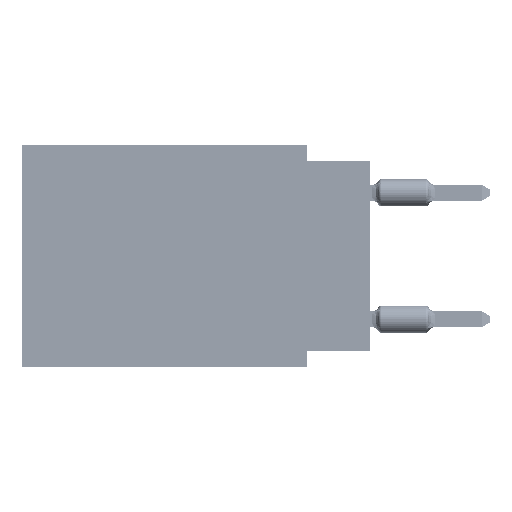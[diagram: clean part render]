
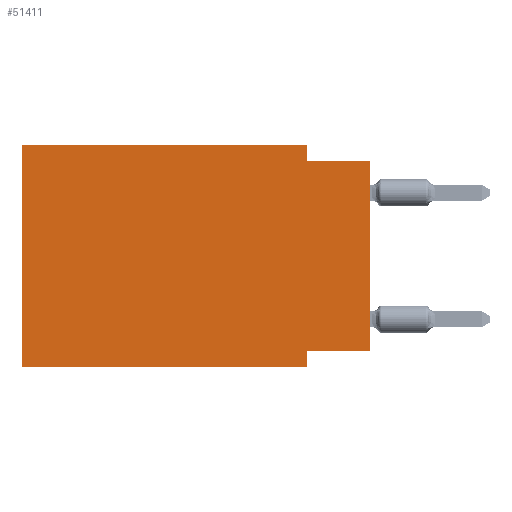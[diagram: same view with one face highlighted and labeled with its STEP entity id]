
A CAD part, left-side view. The second image highlights one B-rep face of the part: STEP entity #51411.
In plain terms, the highlighted planar face has unit normal (-1, 0, 0).
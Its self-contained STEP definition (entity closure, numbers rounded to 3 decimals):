
#2846 = DIRECTION ( 'NONE',  ( 0., 0., -1. ) ) ;
#4109 = DIRECTION ( 'NONE',  ( 0., 0., 1. ) ) ;
#4521 = LINE ( 'NONE', #8218, #76944 ) ;
#4788 = CARTESIAN_POINT ( 'NONE',  ( 0., 0., -0.635 ) ) ;
#6549 = CARTESIAN_POINT ( 'NONE',  ( 0., 2.54, 0. ) ) ;
#6938 = PLANE ( 'NONE',  #75729 ) ;
#8218 = CARTESIAN_POINT ( 'NONE',  ( 0., 2.54, 0. ) ) ;
#8310 = VECTOR ( 'NONE', #4109, 1000. ) ;
#9479 = ORIENTED_EDGE ( 'NONE', *, *, #40379, .T. ) ;
#9956 = VERTEX_POINT ( 'NONE', #65467 ) ;
#10129 = VECTOR ( 'NONE', #35902, 1000. ) ;
#10165 = ORIENTED_EDGE ( 'NONE', *, *, #57154, .F. ) ;
#11423 = VERTEX_POINT ( 'NONE', #36350 ) ;
#12051 = EDGE_CURVE ( 'NONE', #71696, #49729, #40936, .T. ) ;
#18759 = VECTOR ( 'NONE', #71883, 1000. ) ;
#18828 = CARTESIAN_POINT ( 'NONE',  ( 0., 0., 0. ) ) ;
#19589 = LINE ( 'NONE', #58834, #8310 ) ;
#22375 = CARTESIAN_POINT ( 'NONE',  ( 0., 13.97, -8.89 ) ) ;
#23101 = LINE ( 'NONE', #53623, #18759 ) ;
#23820 = VERTEX_POINT ( 'NONE', #47737 ) ;
#26851 = EDGE_CURVE ( 'NONE', #49729, #57755, #4521, .T. ) ;
#28266 = CARTESIAN_POINT ( 'NONE',  ( 0., 13.97, 0. ) ) ;
#31113 = CARTESIAN_POINT ( 'NONE',  ( 0., 13.97, 0. ) ) ;
#32017 = DIRECTION ( 'NONE',  ( 0., -1., 0. ) ) ;
#33629 = CARTESIAN_POINT ( 'NONE',  ( 0., 2.54, -0.635 ) ) ;
#34248 = EDGE_CURVE ( 'NONE', #57755, #11423, #39673, .T. ) ;
#35003 = DIRECTION ( 'NONE',  ( 0., -1., 0. ) ) ;
#35902 = DIRECTION ( 'NONE',  ( 0., 0., 1. ) ) ;
#36350 = CARTESIAN_POINT ( 'NONE',  ( 0., 0., -0.635 ) ) ;
#37305 = LINE ( 'NONE', #38091, #49177 ) ;
#37329 = EDGE_CURVE ( 'NONE', #37973, #60269, #49864, .T. ) ;
#37948 = CARTESIAN_POINT ( 'NONE',  ( 0., 13.97, -8.89 ) ) ;
#37973 = VERTEX_POINT ( 'NONE', #22375 ) ;
#38091 = CARTESIAN_POINT ( 'NONE',  ( 0., 2.54, -8.89 ) ) ;
#38748 = VECTOR ( 'NONE', #40457, 1000. ) ;
#38909 = DIRECTION ( 'NONE',  ( 1., 0., 0. ) ) ;
#39592 = VECTOR ( 'NONE', #35003, 1000. ) ;
#39673 = LINE ( 'NONE', #4788, #38748 ) ;
#40354 = VECTOR ( 'NONE', #32017, 1000. ) ;
#40379 = EDGE_CURVE ( 'NONE', #9956, #11423, #48586, .T. ) ;
#40457 = DIRECTION ( 'NONE',  ( 0., -1., 0. ) ) ;
#40936 = LINE ( 'NONE', #28266, #39592 ) ;
#45199 = ORIENTED_EDGE ( 'NONE', *, *, #26851, .F. ) ;
#46511 = ORIENTED_EDGE ( 'NONE', *, *, #34248, .F. ) ;
#47737 = CARTESIAN_POINT ( 'NONE',  ( 0., 2.54, -8.255 ) ) ;
#48586 = LINE ( 'NONE', #18828, #10129 ) ;
#49177 = VECTOR ( 'NONE', #55575, 1000. ) ;
#49729 = VERTEX_POINT ( 'NONE', #6549 ) ;
#49864 = LINE ( 'NONE', #37948, #40354 ) ;
#50315 = CARTESIAN_POINT ( 'NONE',  ( 0., 13.97, 0. ) ) ;
#51411 = ADVANCED_FACE ( 'NONE', ( #57184 ), #6938, .F. ) ;
#53623 = CARTESIAN_POINT ( 'NONE',  ( 0., 0., -8.255 ) ) ;
#55575 = DIRECTION ( 'NONE',  ( 0., 0., -1. ) ) ;
#57000 = DIRECTION ( 'NONE',  ( 0., 0., -1. ) ) ;
#57065 = EDGE_CURVE ( 'NONE', #9956, #23820, #23101, .T. ) ;
#57154 = EDGE_CURVE ( 'NONE', #23820, #60269, #37305, .T. ) ;
#57184 = FACE_OUTER_BOUND ( 'NONE', #75700, .T. ) ;
#57755 = VERTEX_POINT ( 'NONE', #33629 ) ;
#58834 = CARTESIAN_POINT ( 'NONE',  ( 0., 13.97, 0. ) ) ;
#59504 = ORIENTED_EDGE ( 'NONE', *, *, #12051, .F. ) ;
#60269 = VERTEX_POINT ( 'NONE', #65994 ) ;
#63377 = ORIENTED_EDGE ( 'NONE', *, *, #65640, .F. ) ;
#65467 = CARTESIAN_POINT ( 'NONE',  ( 0., 0., -8.255 ) ) ;
#65640 = EDGE_CURVE ( 'NONE', #37973, #71696, #19589, .T. ) ;
#65994 = CARTESIAN_POINT ( 'NONE',  ( 0., 2.54, -8.89 ) ) ;
#71696 = VERTEX_POINT ( 'NONE', #50315 ) ;
#71883 = DIRECTION ( 'NONE',  ( 0., 1., 0. ) ) ;
#73904 = ORIENTED_EDGE ( 'NONE', *, *, #57065, .F. ) ;
#74302 = ORIENTED_EDGE ( 'NONE', *, *, #37329, .T. ) ;
#75700 = EDGE_LOOP ( 'NONE', ( #9479, #46511, #45199, #59504, #63377, #74302, #10165, #73904 ) ) ;
#75729 = AXIS2_PLACEMENT_3D ( 'NONE', #31113, #38909, #2846 ) ;
#76944 = VECTOR ( 'NONE', #57000, 1000. ) ;
